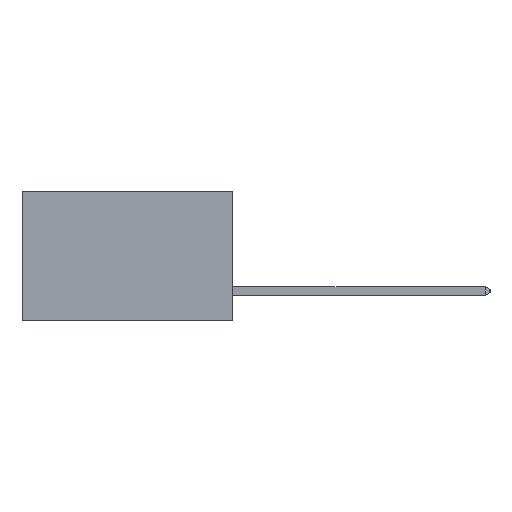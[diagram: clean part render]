
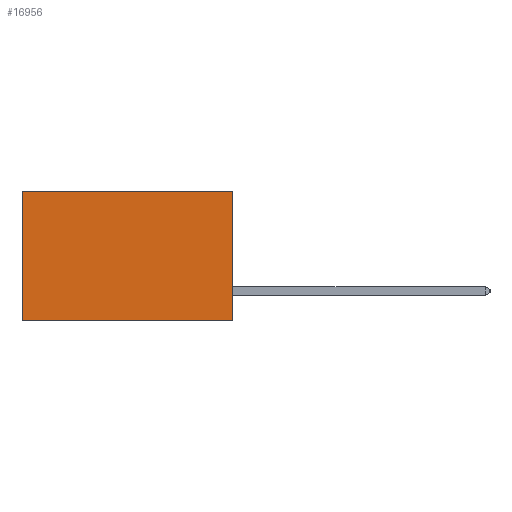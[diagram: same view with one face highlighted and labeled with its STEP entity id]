
A CAD part, left-side view. The second image highlights one B-rep face of the part: STEP entity #16956.
In plain terms, the highlighted planar face has unit normal (-1, 0, 0).
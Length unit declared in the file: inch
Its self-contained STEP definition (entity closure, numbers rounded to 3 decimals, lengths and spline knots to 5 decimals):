
#417 = VERTEX_POINT ( 'NONE', #27084 ) ;
#965 = CARTESIAN_POINT ( 'NONE',  ( 0.2875, 0., 0. ) ) ;
#1329 = DIRECTION ( 'NONE',  ( 0., 0., -1. ) ) ;
#2333 = EDGE_CURVE ( 'NONE', #417, #17634, #10690, .T. ) ;
#3260 = EDGE_CURVE ( 'NONE', #17931, #417, #19623, .T. ) ;
#4362 = CARTESIAN_POINT ( 'NONE',  ( 0.2875, 0.6, 0. ) ) ;
#4756 = CARTESIAN_POINT ( 'NONE',  ( 0.2875, 0., 0. ) ) ;
#4890 = CARTESIAN_POINT ( 'NONE',  ( 0.2875, 0., 0. ) ) ;
#6847 = LINE ( 'NONE', #24514, #17942 ) ;
#8593 = CARTESIAN_POINT ( 'NONE',  ( 0.2875, 0.6, -0.37 ) ) ;
#9347 = DIRECTION ( 'NONE',  ( 1., 0., 0. ) ) ;
#9478 = ORIENTED_EDGE ( 'NONE', *, *, #2333, .F. ) ;
#10690 = LINE ( 'NONE', #21019, #26882 ) ;
#11276 = ORIENTED_EDGE ( 'NONE', *, *, #18848, .T. ) ;
#11473 = ORIENTED_EDGE ( 'NONE', *, *, #13573, .T. ) ;
#13494 = CARTESIAN_POINT ( 'NONE',  ( 0.2875, 0.6, 0. ) ) ;
#13573 = EDGE_CURVE ( 'NONE', #17931, #27239, #6847, .T. ) ;
#13771 = VECTOR ( 'NONE', #1329, 39.37008 ) ;
#14792 = LINE ( 'NONE', #13494, #19276 ) ;
#15722 = DIRECTION ( 'NONE',  ( 0., 0., -1. ) ) ;
#16139 = AXIS2_PLACEMENT_3D ( 'NONE', #4890, #9347, #24776 ) ;
#16956 = ADVANCED_FACE ( 'NONE', ( #25570 ), #26888, .F. ) ;
#17634 = VERTEX_POINT ( 'NONE', #8593 ) ;
#17765 = EDGE_LOOP ( 'NONE', ( #11276, #9478, #20758, #11473 ) ) ;
#17931 = VERTEX_POINT ( 'NONE', #965 ) ;
#17942 = VECTOR ( 'NONE', #26714, 39.37008 ) ;
#18848 = EDGE_CURVE ( 'NONE', #27239, #17634, #14792, .T. ) ;
#19276 = VECTOR ( 'NONE', #15722, 39.37008 ) ;
#19623 = LINE ( 'NONE', #4756, #13771 ) ;
#20758 = ORIENTED_EDGE ( 'NONE', *, *, #3260, .F. ) ;
#21019 = CARTESIAN_POINT ( 'NONE',  ( 0.2875, 0., -0.37 ) ) ;
#23031 = DIRECTION ( 'NONE',  ( 0., 1., 0. ) ) ;
#24514 = CARTESIAN_POINT ( 'NONE',  ( 0.2875, 0., 0. ) ) ;
#24776 = DIRECTION ( 'NONE',  ( 0., 0., -1. ) ) ;
#25570 = FACE_OUTER_BOUND ( 'NONE', #17765, .T. ) ;
#26714 = DIRECTION ( 'NONE',  ( 0., 1., 0. ) ) ;
#26882 = VECTOR ( 'NONE', #23031, 39.37008 ) ;
#26888 = PLANE ( 'NONE',  #16139 ) ;
#27084 = CARTESIAN_POINT ( 'NONE',  ( 0.2875, 0., -0.37 ) ) ;
#27239 = VERTEX_POINT ( 'NONE', #4362 ) ;
